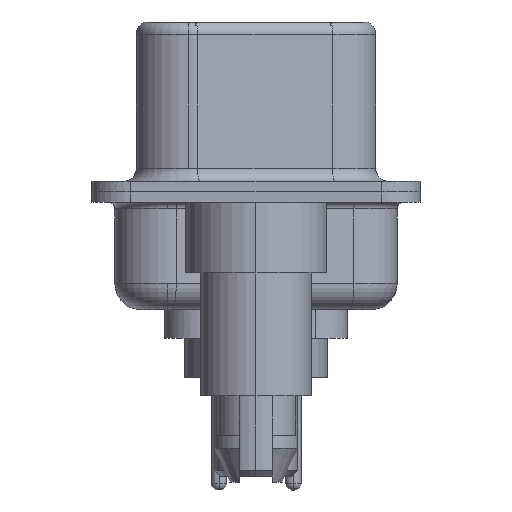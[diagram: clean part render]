
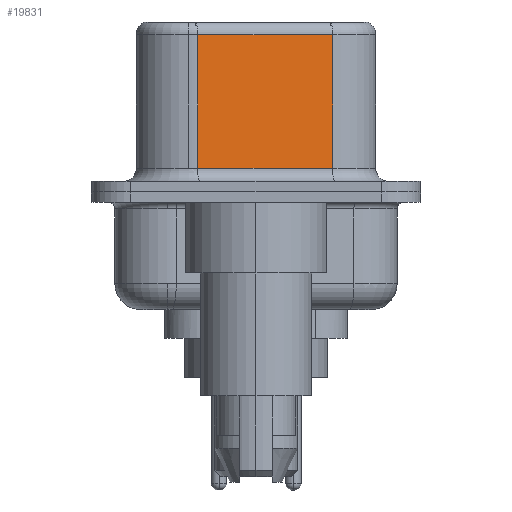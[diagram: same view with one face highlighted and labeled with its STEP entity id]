
A CAD part, left-side view. The second image highlights one B-rep face of the part: STEP entity #19831.
In plain terms, the highlighted planar face has unit normal (-0.985, -0.174, 0).
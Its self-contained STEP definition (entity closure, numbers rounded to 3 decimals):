
#368 = ORIENTED_EDGE ( 'NONE', *, *, #378, .F. ) ;
#378 = EDGE_CURVE ( 'NONE', #11166, #19167, #11397, .T. ) ;
#2014 = VECTOR ( 'NONE', #14416, 1000. ) ;
#2335 = CARTESIAN_POINT ( 'NONE',  ( 3.67, 2.233, 6.02 ) ) ;
#2727 = VERTEX_POINT ( 'NONE', #2335 ) ;
#2851 = CARTESIAN_POINT ( 'NONE',  ( 4.58, -2.927, 0.9 ) ) ;
#3391 = VERTEX_POINT ( 'NONE', #18213 ) ;
#3920 = PLANE ( 'NONE',  #24288 ) ;
#4792 = EDGE_CURVE ( 'NONE', #3391, #19167, #6321, .T. ) ;
#4924 = EDGE_CURVE ( 'NONE', #2727, #3391, #9118, .T. ) ;
#5966 = DIRECTION ( 'NONE',  ( 0.985, 0.174, 0. ) ) ;
#6321 = LINE ( 'NONE', #2851, #11699 ) ;
#7726 = CARTESIAN_POINT ( 'NONE',  ( 4.58, -2.927, 6.52 ) ) ;
#8532 = ORIENTED_EDGE ( 'NONE', *, *, #4924, .T. ) ;
#9118 = LINE ( 'NONE', #23281, #24131 ) ;
#10021 = CARTESIAN_POINT ( 'NONE',  ( 4.58, -2.927, 0.9 ) ) ;
#10381 = FACE_OUTER_BOUND ( 'NONE', #13306, .T. ) ;
#11166 = VERTEX_POINT ( 'NONE', #17266 ) ;
#11397 = LINE ( 'NONE', #26471, #22273 ) ;
#11699 = VECTOR ( 'NONE', #17083, 1000. ) ;
#13306 = EDGE_LOOP ( 'NONE', ( #368, #24900, #8532, #17071 ) ) ;
#14194 = DIRECTION ( 'NONE',  ( 0., 0., -1. ) ) ;
#14416 = DIRECTION ( 'NONE',  ( -0.174, 0.985, 0. ) ) ;
#16698 = EDGE_CURVE ( 'NONE', #11166, #2727, #24349, .T. ) ;
#17071 = ORIENTED_EDGE ( 'NONE', *, *, #4792, .T. ) ;
#17083 = DIRECTION ( 'NONE',  ( 0.174, -0.985, 0. ) ) ;
#17266 = CARTESIAN_POINT ( 'NONE',  ( 4.58, -2.927, 6.02 ) ) ;
#18213 = CARTESIAN_POINT ( 'NONE',  ( 3.67, 2.233, 0.9 ) ) ;
#19167 = VERTEX_POINT ( 'NONE', #10021 ) ;
#19831 = ADVANCED_FACE ( 'NONE', ( #10381 ), #3920, .F. ) ;
#20178 = DIRECTION ( 'NONE',  ( -0.174, 0.985, 0. ) ) ;
#20397 = CARTESIAN_POINT ( 'NONE',  ( 4.58, -2.927, 6.02 ) ) ;
#22273 = VECTOR ( 'NONE', #25020, 1000. ) ;
#23281 = CARTESIAN_POINT ( 'NONE',  ( 3.67, 2.233, 6.52 ) ) ;
#24131 = VECTOR ( 'NONE', #14194, 1000. ) ;
#24288 = AXIS2_PLACEMENT_3D ( 'NONE', #7726, #5966, #20178 ) ;
#24349 = LINE ( 'NONE', #20397, #2014 ) ;
#24900 = ORIENTED_EDGE ( 'NONE', *, *, #16698, .T. ) ;
#25020 = DIRECTION ( 'NONE',  ( 0., 0., -1. ) ) ;
#26471 = CARTESIAN_POINT ( 'NONE',  ( 4.58, -2.927, 6.52 ) ) ;
